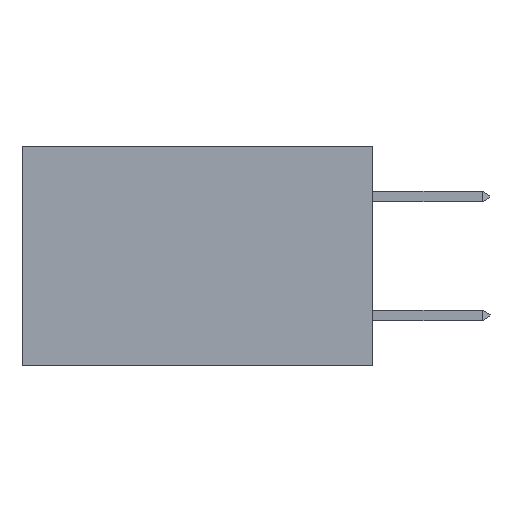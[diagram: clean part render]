
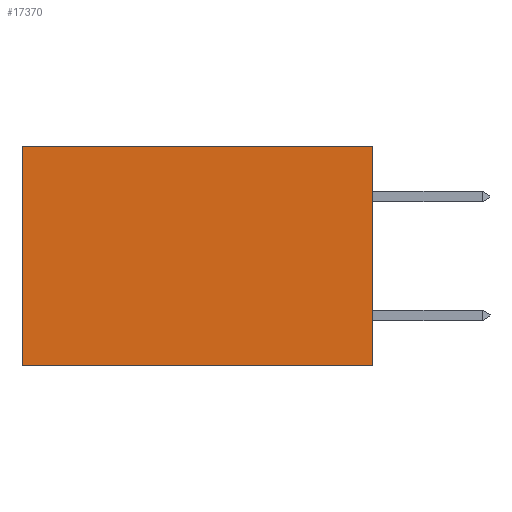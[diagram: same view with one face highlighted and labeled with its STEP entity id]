
A CAD part, left-side view. The second image highlights one B-rep face of the part: STEP entity #17370.
In plain terms, the highlighted planar face has unit normal (-1, 0, 0).
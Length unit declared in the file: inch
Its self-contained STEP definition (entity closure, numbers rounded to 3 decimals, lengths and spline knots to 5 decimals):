
#280 = EDGE_CURVE ( 'NONE', #27583, #10288, #15546, .T. ) ;
#791 = AXIS2_PLACEMENT_3D ( 'NONE', #7378, #26152, #12122 ) ;
#1904 = LINE ( 'NONE', #25815, #13736 ) ;
#3751 = VECTOR ( 'NONE', #21681, 39.37008 ) ;
#4759 = CARTESIAN_POINT ( 'NONE',  ( 0.277, 0., -0.37 ) ) ;
#5114 = ORIENTED_EDGE ( 'NONE', *, *, #13642, .F. ) ;
#5357 = VERTEX_POINT ( 'NONE', #15959 ) ;
#6719 = VERTEX_POINT ( 'NONE', #19175 ) ;
#7378 = CARTESIAN_POINT ( 'NONE',  ( 0.277, 0., -0.37 ) ) ;
#7629 = VECTOR ( 'NONE', #12359, 39.37008 ) ;
#7631 = CARTESIAN_POINT ( 'NONE',  ( 0.277, 0., -0.37 ) ) ;
#9403 = DIRECTION ( 'NONE',  ( 0., 0., -1. ) ) ;
#9516 = VECTOR ( 'NONE', #17710, 39.37008 ) ;
#10288 = VERTEX_POINT ( 'NONE', #4759 ) ;
#10572 = ORIENTED_EDGE ( 'NONE', *, *, #280, .F. ) ;
#10616 = CARTESIAN_POINT ( 'NONE',  ( 0.277, 0., 0. ) ) ;
#12122 = DIRECTION ( 'NONE',  ( 0., 0., -1. ) ) ;
#12359 = DIRECTION ( 'NONE',  ( 0., 1., 0. ) ) ;
#13642 = EDGE_CURVE ( 'NONE', #10288, #5357, #13888, .T. ) ;
#13736 = VECTOR ( 'NONE', #9403, 39.37008 ) ;
#13888 = LINE ( 'NONE', #7631, #7629 ) ;
#15184 = ORIENTED_EDGE ( 'NONE', *, *, #21802, .T. ) ;
#15546 = LINE ( 'NONE', #19542, #3751 ) ;
#15757 = LINE ( 'NONE', #10616, #9516 ) ;
#15959 = CARTESIAN_POINT ( 'NONE',  ( 0.277, 0.59, -0.37 ) ) ;
#17370 = ADVANCED_FACE ( 'NONE', ( #25892 ), #21440, .F. ) ;
#17710 = DIRECTION ( 'NONE',  ( 0., 1., 0. ) ) ;
#18361 = EDGE_LOOP ( 'NONE', ( #22650, #5114, #10572, #15184 ) ) ;
#19175 = CARTESIAN_POINT ( 'NONE',  ( 0.277, 0.59, 0. ) ) ;
#19542 = CARTESIAN_POINT ( 'NONE',  ( 0.277, 0., -0.37 ) ) ;
#21440 = PLANE ( 'NONE',  #791 ) ;
#21681 = DIRECTION ( 'NONE',  ( 0., 0., -1. ) ) ;
#21802 = EDGE_CURVE ( 'NONE', #27583, #6719, #15757, .T. ) ;
#22650 = ORIENTED_EDGE ( 'NONE', *, *, #28521, .T. ) ;
#25815 = CARTESIAN_POINT ( 'NONE',  ( 0.277, 0.59, -0.37 ) ) ;
#25892 = FACE_OUTER_BOUND ( 'NONE', #18361, .T. ) ;
#26152 = DIRECTION ( 'NONE',  ( 1., 0., 0. ) ) ;
#27583 = VERTEX_POINT ( 'NONE', #29892 ) ;
#28521 = EDGE_CURVE ( 'NONE', #6719, #5357, #1904, .T. ) ;
#29892 = CARTESIAN_POINT ( 'NONE',  ( 0.277, 0., 0. ) ) ;
